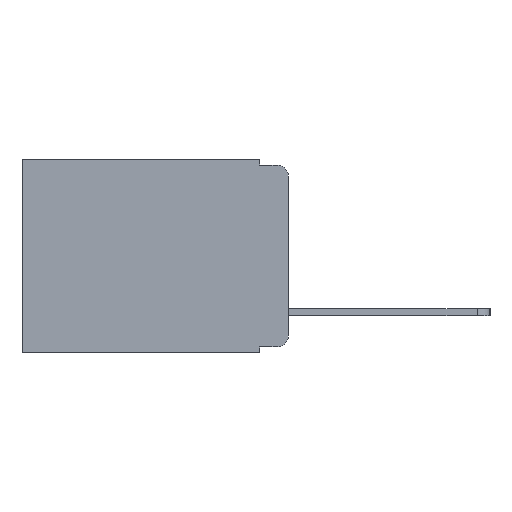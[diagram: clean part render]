
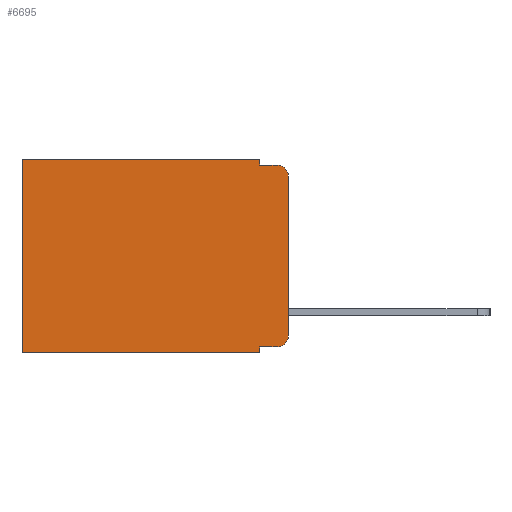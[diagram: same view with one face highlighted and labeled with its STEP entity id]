
A CAD part, left-side view. The second image highlights one B-rep face of the part: STEP entity #6695.
In plain terms, the highlighted planar face has unit normal (-1, 0, 0).
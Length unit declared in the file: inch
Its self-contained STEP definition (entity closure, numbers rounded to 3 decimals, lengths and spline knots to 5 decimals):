
#66 = LINE ( 'NONE', #3473, #10886 ) ;
#143 = ORIENTED_EDGE ( 'NONE', *, *, #7132, .T. ) ;
#299 = DIRECTION ( 'NONE',  ( 0., 0., -1. ) ) ;
#357 = VECTOR ( 'NONE', #9961, 39.37008 ) ;
#522 = CARTESIAN_POINT ( 'NONE',  ( 0.298, 0.051, 0. ) ) ;
#1107 = VERTEX_POINT ( 'NONE', #10425 ) ;
#1233 = CARTESIAN_POINT ( 'NONE',  ( 0.298, 0., -0.03 ) ) ;
#1293 = DIRECTION ( 'NONE',  ( 0., 1., 0. ) ) ;
#1339 = CIRCLE ( 'NONE', #3825, 0.02 ) ;
#1411 = FACE_OUTER_BOUND ( 'NONE', #3226, .T. ) ;
#1608 = PLANE ( 'NONE',  #10965 ) ;
#1757 = VERTEX_POINT ( 'NONE', #8414 ) ;
#1914 = VECTOR ( 'NONE', #4887, 39.37008 ) ;
#2001 = VERTEX_POINT ( 'NONE', #7520 ) ;
#2160 = LINE ( 'NONE', #3198, #8416 ) ;
#2324 = CIRCLE ( 'NONE', #4064, 0.02 ) ;
#2570 = EDGE_CURVE ( 'NONE', #1757, #6882, #10597, .T. ) ;
#2641 = LINE ( 'NONE', #7585, #9069 ) ;
#2682 = ORIENTED_EDGE ( 'NONE', *, *, #2570, .T. ) ;
#2701 = CARTESIAN_POINT ( 'NONE',  ( 0.298, 0.051, -0.333 ) ) ;
#2837 = CARTESIAN_POINT ( 'NONE',  ( 0.298, 0.473, -0.343 ) ) ;
#2938 = CARTESIAN_POINT ( 'NONE',  ( 0.298, 0.473, 0. ) ) ;
#3198 = CARTESIAN_POINT ( 'NONE',  ( 0.298, 0., -0.343 ) ) ;
#3226 = EDGE_LOOP ( 'NONE', ( #3389, #6186, #3818, #7915, #2682, #143, #9729, #3673, #6627, #3800 ) ) ;
#3389 = ORIENTED_EDGE ( 'NONE', *, *, #4001, .F. ) ;
#3434 = DIRECTION ( 'NONE',  ( 0., 0., -1. ) ) ;
#3473 = CARTESIAN_POINT ( 'NONE',  ( 0.298, 0.051, 0. ) ) ;
#3523 = DIRECTION ( 'NONE',  ( 1., 0., 0. ) ) ;
#3673 = ORIENTED_EDGE ( 'NONE', *, *, #7118, .F. ) ;
#3800 = ORIENTED_EDGE ( 'NONE', *, *, #6979, .T. ) ;
#3818 = ORIENTED_EDGE ( 'NONE', *, *, #8104, .F. ) ;
#3825 = AXIS2_PLACEMENT_3D ( 'NONE', #5329, #10902, #6154 ) ;
#3853 = VERTEX_POINT ( 'NONE', #9758 ) ;
#4001 = EDGE_CURVE ( 'NONE', #6505, #3853, #10808, .T. ) ;
#4064 = AXIS2_PLACEMENT_3D ( 'NONE', #10540, #5781, #299 ) ;
#4860 = CARTESIAN_POINT ( 'NONE',  ( 0.298, 0., 0. ) ) ;
#4887 = DIRECTION ( 'NONE',  ( 0., 0., -1. ) ) ;
#5191 = DIRECTION ( 'NONE',  ( 0., 0., -1. ) ) ;
#5329 = CARTESIAN_POINT ( 'NONE',  ( 0.298, 0.02, -0.03 ) ) ;
#5431 = DIRECTION ( 'NONE',  ( 0., 1., 0. ) ) ;
#5765 = VERTEX_POINT ( 'NONE', #2837 ) ;
#5781 = DIRECTION ( 'NONE',  ( -1., 0., 0. ) ) ;
#5904 = VECTOR ( 'NONE', #8311, 39.37008 ) ;
#6154 = DIRECTION ( 'NONE',  ( 0., 0., -1. ) ) ;
#6186 = ORIENTED_EDGE ( 'NONE', *, *, #9764, .T. ) ;
#6258 = CARTESIAN_POINT ( 'NONE',  ( 0.298, 0.051, -0.01 ) ) ;
#6505 = VERTEX_POINT ( 'NONE', #1233 ) ;
#6597 = VERTEX_POINT ( 'NONE', #9905 ) ;
#6627 = ORIENTED_EDGE ( 'NONE', *, *, #7048, .T. ) ;
#6695 = ADVANCED_FACE ( 'NONE', ( #1411 ), #1608, .F. ) ;
#6882 = VERTEX_POINT ( 'NONE', #2938 ) ;
#6979 = EDGE_CURVE ( 'NONE', #2001, #3853, #2324, .T. ) ;
#7048 = EDGE_CURVE ( 'NONE', #9814, #2001, #7763, .T. ) ;
#7080 = DIRECTION ( 'NONE',  ( 0., -1., 0. ) ) ;
#7118 = EDGE_CURVE ( 'NONE', #9814, #1107, #9559, .T. ) ;
#7132 = EDGE_CURVE ( 'NONE', #6882, #5765, #2641, .T. ) ;
#7154 = EDGE_CURVE ( 'NONE', #1757, #7661, #66, .T. ) ;
#7160 = CARTESIAN_POINT ( 'NONE',  ( 0.298, 0.051, -0.01 ) ) ;
#7520 = CARTESIAN_POINT ( 'NONE',  ( 0.298, 0.02, -0.333 ) ) ;
#7585 = CARTESIAN_POINT ( 'NONE',  ( 0.298, 0.473, 0. ) ) ;
#7658 = CARTESIAN_POINT ( 'NONE',  ( 0.298, 0., 0. ) ) ;
#7661 = VERTEX_POINT ( 'NONE', #7160 ) ;
#7763 = LINE ( 'NONE', #10638, #5904 ) ;
#7808 = EDGE_CURVE ( 'NONE', #1107, #5765, #2160, .T. ) ;
#7915 = ORIENTED_EDGE ( 'NONE', *, *, #7154, .F. ) ;
#7994 = VECTOR ( 'NONE', #5431, 39.37008 ) ;
#8104 = EDGE_CURVE ( 'NONE', #7661, #6597, #9163, .T. ) ;
#8311 = DIRECTION ( 'NONE',  ( 0., -1., 0. ) ) ;
#8414 = CARTESIAN_POINT ( 'NONE',  ( 0.298, 0.051, 0. ) ) ;
#8416 = VECTOR ( 'NONE', #1293, 39.37008 ) ;
#8916 = VECTOR ( 'NONE', #7080, 39.37008 ) ;
#9069 = VECTOR ( 'NONE', #5191, 39.37008 ) ;
#9163 = LINE ( 'NONE', #6258, #8916 ) ;
#9297 = DIRECTION ( 'NONE',  ( 0., 0., -1. ) ) ;
#9559 = LINE ( 'NONE', #522, #357 ) ;
#9729 = ORIENTED_EDGE ( 'NONE', *, *, #7808, .F. ) ;
#9758 = CARTESIAN_POINT ( 'NONE',  ( 0.298, 0., -0.313 ) ) ;
#9764 = EDGE_CURVE ( 'NONE', #6505, #6597, #1339, .T. ) ;
#9814 = VERTEX_POINT ( 'NONE', #2701 ) ;
#9905 = CARTESIAN_POINT ( 'NONE',  ( 0.298, 0.02, -0.01 ) ) ;
#9961 = DIRECTION ( 'NONE',  ( 0., 0., -1. ) ) ;
#10004 = CARTESIAN_POINT ( 'NONE',  ( 0.298, 0., 0. ) ) ;
#10425 = CARTESIAN_POINT ( 'NONE',  ( 0.298, 0.051, -0.343 ) ) ;
#10540 = CARTESIAN_POINT ( 'NONE',  ( 0.298, 0.02, -0.313 ) ) ;
#10597 = LINE ( 'NONE', #10004, #7994 ) ;
#10638 = CARTESIAN_POINT ( 'NONE',  ( 0.298, 0.051, -0.333 ) ) ;
#10808 = LINE ( 'NONE', #4860, #1914 ) ;
#10886 = VECTOR ( 'NONE', #3434, 39.37008 ) ;
#10902 = DIRECTION ( 'NONE',  ( -1., 0., 0. ) ) ;
#10965 = AXIS2_PLACEMENT_3D ( 'NONE', #7658, #3523, #9297 ) ;
